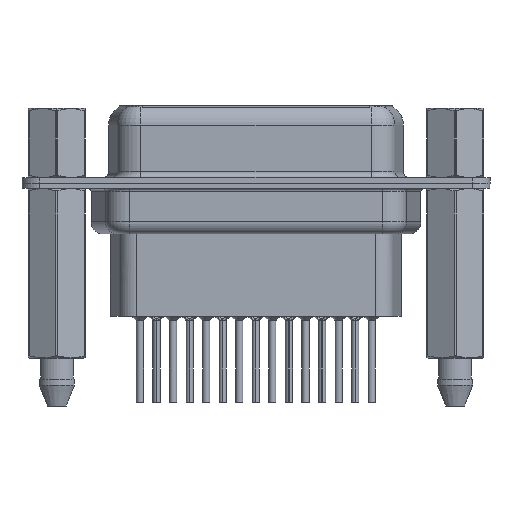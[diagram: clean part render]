
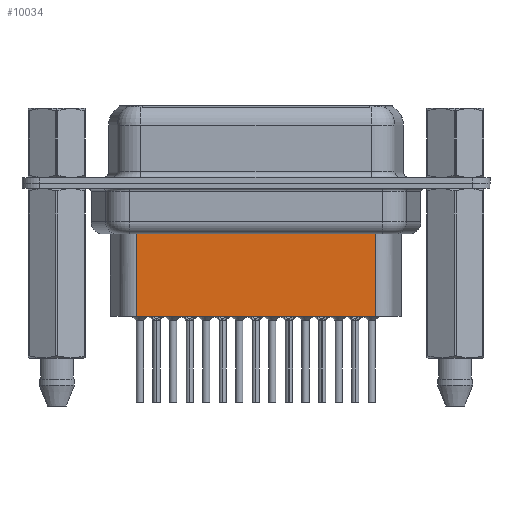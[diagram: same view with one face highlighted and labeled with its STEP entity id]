
A CAD part, front view. The second image highlights one B-rep face of the part: STEP entity #10034.
In plain terms, the highlighted planar face has unit normal (0, -1, 0).
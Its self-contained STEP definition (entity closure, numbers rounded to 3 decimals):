
#337 = ORIENTED_EDGE ( 'NONE', *, *, #25818, .F. ) ;
#1516 = DIRECTION ( 'NONE',  ( 0., -1., 0. ) ) ;
#2304 = DIRECTION ( 'NONE',  ( -1., 0., 0. ) ) ;
#2714 = LINE ( 'NONE', #21491, #17866 ) ;
#3578 = ORIENTED_EDGE ( 'NONE', *, *, #11379, .F. ) ;
#4371 = CARTESIAN_POINT ( 'NONE',  ( 6.434, -3.5, -4.097 ) ) ;
#5467 = DIRECTION ( 'NONE',  ( 1., 0., 0. ) ) ;
#5620 = EDGE_LOOP ( 'NONE', ( #3578, #10183, #11464, #337 ) ) ;
#7094 = DIRECTION ( 'NONE',  ( 0., 0., -1. ) ) ;
#10034 = ADVANCED_FACE ( 'NONE', ( #26189 ), #16961, .T. ) ;
#10183 = ORIENTED_EDGE ( 'NONE', *, *, #11664, .T. ) ;
#11379 = EDGE_CURVE ( 'NONE', #15388, #20750, #16927, .T. ) ;
#11464 = ORIENTED_EDGE ( 'NONE', *, *, #29852, .T. ) ;
#11664 = EDGE_CURVE ( 'NONE', #15388, #12997, #27341, .T. ) ;
#12997 = VERTEX_POINT ( 'NONE', #21186 ) ;
#15388 = VERTEX_POINT ( 'NONE', #19039 ) ;
#15782 = CARTESIAN_POINT ( 'NONE',  ( 6.681, -3.5, -11.15 ) ) ;
#16927 = LINE ( 'NONE', #21337, #27354 ) ;
#16961 = PLANE ( 'NONE',  #25353 ) ;
#17866 = VECTOR ( 'NONE', #21627, 1000. ) ;
#19039 = CARTESIAN_POINT ( 'NONE',  ( 26.619, -3.5, -4.097 ) ) ;
#20481 = VECTOR ( 'NONE', #2304, 1000. ) ;
#20750 = VERTEX_POINT ( 'NONE', #21069 ) ;
#21069 = CARTESIAN_POINT ( 'NONE',  ( 26.619, -3.5, -11.15 ) ) ;
#21186 = CARTESIAN_POINT ( 'NONE',  ( 6.681, -3.5, -4.097 ) ) ;
#21337 = CARTESIAN_POINT ( 'NONE',  ( 26.619, -3.5, -3.1 ) ) ;
#21491 = CARTESIAN_POINT ( 'NONE',  ( 6.681, -3.5, -3.1 ) ) ;
#21627 = DIRECTION ( 'NONE',  ( 0., 0., -1. ) ) ;
#22252 = CARTESIAN_POINT ( 'NONE',  ( 6.681, -3.5, -3.1 ) ) ;
#25078 = DIRECTION ( 'NONE',  ( -1., 0., 0. ) ) ;
#25353 = AXIS2_PLACEMENT_3D ( 'NONE', #22252, #1516, #5467 ) ;
#25818 = EDGE_CURVE ( 'NONE', #20750, #28871, #29556, .T. ) ;
#26189 = FACE_OUTER_BOUND ( 'NONE', #5620, .T. ) ;
#27341 = LINE ( 'NONE', #4371, #27825 ) ;
#27354 = VECTOR ( 'NONE', #7094, 1000. ) ;
#27825 = VECTOR ( 'NONE', #25078, 1000. ) ;
#28310 = CARTESIAN_POINT ( 'NONE',  ( 6.681, -3.5, -11.15 ) ) ;
#28871 = VERTEX_POINT ( 'NONE', #28310 ) ;
#29556 = LINE ( 'NONE', #15782, #20481 ) ;
#29852 = EDGE_CURVE ( 'NONE', #12997, #28871, #2714, .T. ) ;
